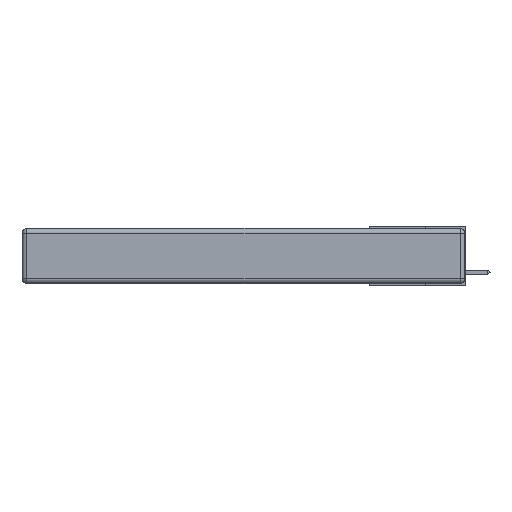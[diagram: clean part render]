
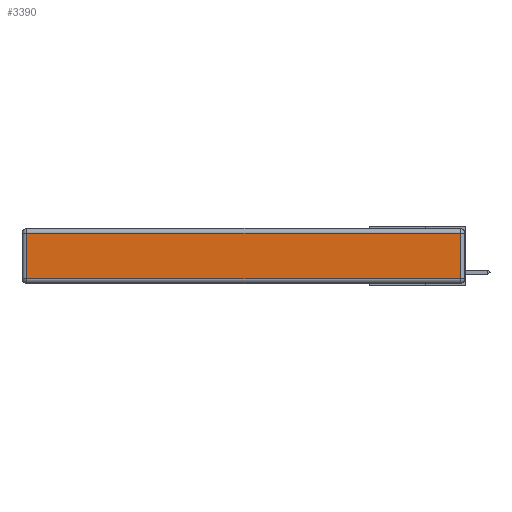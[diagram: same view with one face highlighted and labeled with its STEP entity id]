
A CAD part, left-side view. The second image highlights one B-rep face of the part: STEP entity #3390.
In plain terms, the highlighted planar face has unit normal (-1, 0, 0).
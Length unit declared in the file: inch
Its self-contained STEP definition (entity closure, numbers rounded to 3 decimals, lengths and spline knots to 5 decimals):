
#654 = VECTOR ( 'NONE', #3337, 39.37008 ) ;
#691 = LINE ( 'NONE', #21285, #6119 ) ;
#1350 = VERTEX_POINT ( 'NONE', #11768 ) ;
#1870 = EDGE_CURVE ( 'NONE', #22248, #22105, #19877, .T. ) ;
#2023 = LINE ( 'NONE', #11710, #11033 ) ;
#3337 = DIRECTION ( 'NONE',  ( 0., -1., 0. ) ) ;
#3390 = ADVANCED_FACE ( 'NONE', ( #4885 ), #24573, .T. ) ;
#3618 = EDGE_LOOP ( 'NONE', ( #14287, #6725, #16578, #13385 ) ) ;
#3781 = DIRECTION ( 'NONE',  ( 0., 0., -1. ) ) ;
#4885 = FACE_OUTER_BOUND ( 'NONE', #3618, .T. ) ;
#5627 = CARTESIAN_POINT ( 'NONE',  ( 0., 2.72, -0.313 ) ) ;
#5794 = LINE ( 'NONE', #24309, #654 ) ;
#6119 = VECTOR ( 'NONE', #13731, 39.37008 ) ;
#6725 = ORIENTED_EDGE ( 'NONE', *, *, #15823, .T. ) ;
#7213 = DIRECTION ( 'NONE',  ( -1., 0., 0. ) ) ;
#7482 = EDGE_CURVE ( 'NONE', #22105, #19481, #5794, .T. ) ;
#7743 = CARTESIAN_POINT ( 'NONE',  ( 0., 2.72, -0.343 ) ) ;
#11033 = VECTOR ( 'NONE', #21975, 39.37008 ) ;
#11710 = CARTESIAN_POINT ( 'NONE',  ( 0., 2.75, -0.03 ) ) ;
#11768 = CARTESIAN_POINT ( 'NONE',  ( 0., 0.03, -0.03 ) ) ;
#11915 = CARTESIAN_POINT ( 'NONE',  ( 0., 0.03, -0.313 ) ) ;
#13385 = ORIENTED_EDGE ( 'NONE', *, *, #1870, .T. ) ;
#13581 = EDGE_CURVE ( 'NONE', #1350, #22248, #2023, .T. ) ;
#13731 = DIRECTION ( 'NONE',  ( 0., 0., 1. ) ) ;
#14287 = ORIENTED_EDGE ( 'NONE', *, *, #7482, .T. ) ;
#14828 = VECTOR ( 'NONE', #3781, 39.37008 ) ;
#15823 = EDGE_CURVE ( 'NONE', #19481, #1350, #691, .T. ) ;
#16578 = ORIENTED_EDGE ( 'NONE', *, *, #13581, .T. ) ;
#18421 = CARTESIAN_POINT ( 'NONE',  ( 0., 2.72, -0.03 ) ) ;
#19481 = VERTEX_POINT ( 'NONE', #11915 ) ;
#19877 = LINE ( 'NONE', #7743, #14828 ) ;
#21285 = CARTESIAN_POINT ( 'NONE',  ( 0., 0.03, -0.343 ) ) ;
#21975 = DIRECTION ( 'NONE',  ( 0., 1., 0. ) ) ;
#22105 = VERTEX_POINT ( 'NONE', #5627 ) ;
#22240 = AXIS2_PLACEMENT_3D ( 'NONE', #24484, #7213, #22619 ) ;
#22248 = VERTEX_POINT ( 'NONE', #18421 ) ;
#22619 = DIRECTION ( 'NONE',  ( 0., 0., 1. ) ) ;
#24309 = CARTESIAN_POINT ( 'NONE',  ( 0., 0., -0.313 ) ) ;
#24484 = CARTESIAN_POINT ( 'NONE',  ( 0., 0., -0.343 ) ) ;
#24573 = PLANE ( 'NONE',  #22240 ) ;
